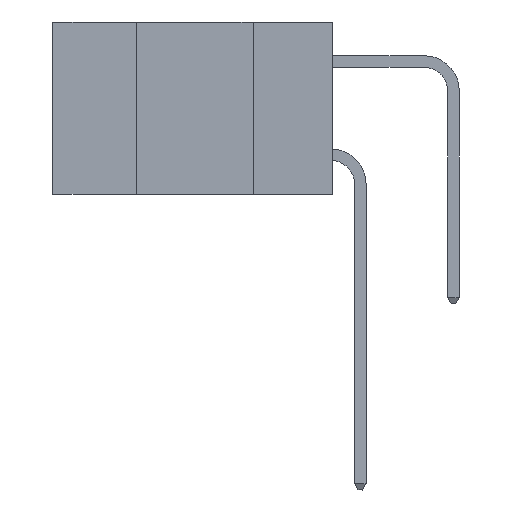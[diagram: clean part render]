
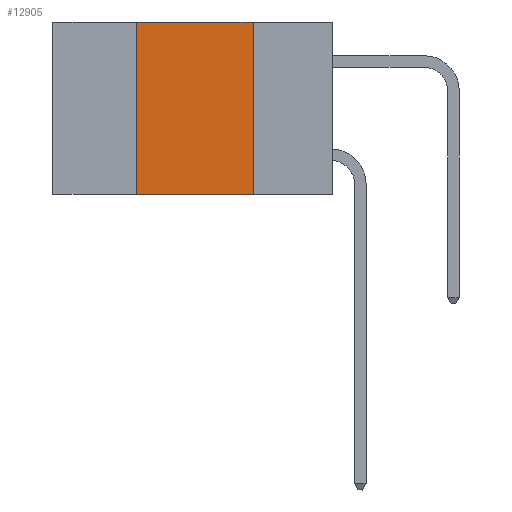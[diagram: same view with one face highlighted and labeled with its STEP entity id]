
A CAD part, left-side view. The second image highlights one B-rep face of the part: STEP entity #12905.
In plain terms, the highlighted planar face has unit normal (-1, 0, 0).
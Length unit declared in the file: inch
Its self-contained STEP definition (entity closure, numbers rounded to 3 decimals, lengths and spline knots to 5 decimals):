
#951 = DIRECTION ( 'NONE',  ( 1., 0., 0. ) ) ;
#1039 = VECTOR ( 'NONE', #4883, 39.37008 ) ;
#1649 = AXIS2_PLACEMENT_3D ( 'NONE', #6586, #951, #10834 ) ;
#1658 = DIRECTION ( 'NONE',  ( 0., -1., 0. ) ) ;
#1736 = CARTESIAN_POINT ( 'NONE',  ( 0., 0.6, -0.37 ) ) ;
#2010 = ORIENTED_EDGE ( 'NONE', *, *, #12747, .F. ) ;
#2043 = VERTEX_POINT ( 'NONE', #5580 ) ;
#3607 = VECTOR ( 'NONE', #1658, 39.37008 ) ;
#4807 = LINE ( 'NONE', #7718, #1039 ) ;
#4883 = DIRECTION ( 'NONE',  ( 0., 0., 1. ) ) ;
#5314 = VERTEX_POINT ( 'NONE', #5355 ) ;
#5355 = CARTESIAN_POINT ( 'NONE',  ( 0., 0.17, -0.37 ) ) ;
#5580 = CARTESIAN_POINT ( 'NONE',  ( 0., 0.42, 0. ) ) ;
#5619 = VERTEX_POINT ( 'NONE', #6370 ) ;
#6267 = CARTESIAN_POINT ( 'NONE',  ( 0., 0.6, 0. ) ) ;
#6335 = VECTOR ( 'NONE', #14590, 39.37008 ) ;
#6370 = CARTESIAN_POINT ( 'NONE',  ( 0., 0.17, 0. ) ) ;
#6471 = ORIENTED_EDGE ( 'NONE', *, *, #10813, .T. ) ;
#6586 = CARTESIAN_POINT ( 'NONE',  ( 0., 0.6, 0. ) ) ;
#7379 = LINE ( 'NONE', #1736, #3607 ) ;
#7718 = CARTESIAN_POINT ( 'NONE',  ( 0., 0.42, 0. ) ) ;
#8269 = VERTEX_POINT ( 'NONE', #8710 ) ;
#8445 = EDGE_CURVE ( 'NONE', #8269, #2043, #4807, .T. ) ;
#8710 = CARTESIAN_POINT ( 'NONE',  ( 0., 0.42, -0.37 ) ) ;
#9854 = FACE_OUTER_BOUND ( 'NONE', #17677, .T. ) ;
#10090 = LINE ( 'NONE', #11773, #6335 ) ;
#10813 = EDGE_CURVE ( 'NONE', #8269, #5314, #7379, .T. ) ;
#10834 = DIRECTION ( 'NONE',  ( 0., 0., -1. ) ) ;
#11174 = VECTOR ( 'NONE', #14768, 39.37008 ) ;
#11303 = ORIENTED_EDGE ( 'NONE', *, *, #13289, .F. ) ;
#11617 = LINE ( 'NONE', #6267, #11174 ) ;
#11773 = CARTESIAN_POINT ( 'NONE',  ( 0., 0.17, 0. ) ) ;
#12747 = EDGE_CURVE ( 'NONE', #5619, #5314, #10090, .T. ) ;
#12905 = ADVANCED_FACE ( 'NONE', ( #9854 ), #17915, .F. ) ;
#13289 = EDGE_CURVE ( 'NONE', #2043, #5619, #11617, .T. ) ;
#13487 = ORIENTED_EDGE ( 'NONE', *, *, #8445, .F. ) ;
#14590 = DIRECTION ( 'NONE',  ( 0., 0., -1. ) ) ;
#14768 = DIRECTION ( 'NONE',  ( 0., -1., 0. ) ) ;
#17677 = EDGE_LOOP ( 'NONE', ( #2010, #11303, #13487, #6471 ) ) ;
#17915 = PLANE ( 'NONE',  #1649 ) ;
